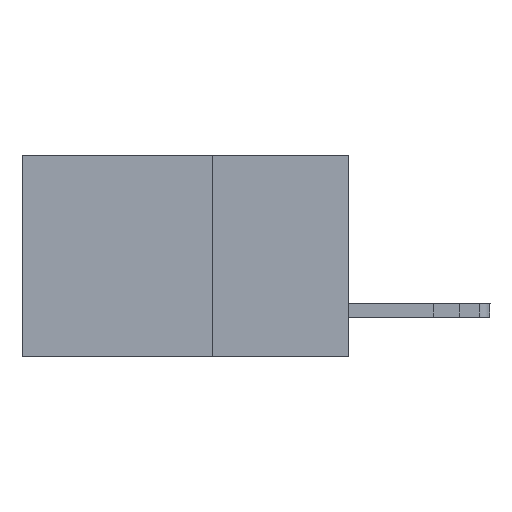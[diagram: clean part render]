
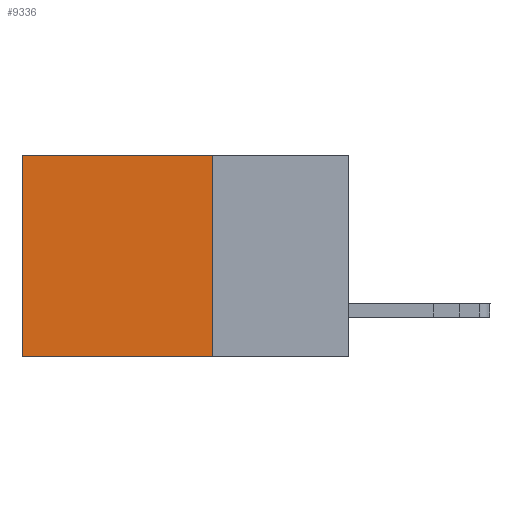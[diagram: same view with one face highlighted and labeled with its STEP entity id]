
A CAD part, left-side view. The second image highlights one B-rep face of the part: STEP entity #9336.
In plain terms, the highlighted planar face has unit normal (-1, 0, 0).
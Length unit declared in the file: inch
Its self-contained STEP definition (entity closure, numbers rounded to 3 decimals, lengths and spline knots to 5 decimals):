
#306 = LINE ( 'NONE', #15764, #18215 ) ;
#2104 = VECTOR ( 'NONE', #7133, 39.37008 ) ;
#2368 = LINE ( 'NONE', #3701, #2104 ) ;
#3596 = DIRECTION ( 'NONE',  ( 0., 1., 0. ) ) ;
#3701 = CARTESIAN_POINT ( 'NONE',  ( 0.298, 0.6, 0. ) ) ;
#3833 = AXIS2_PLACEMENT_3D ( 'NONE', #8523, #11875, #13608 ) ;
#5139 = EDGE_CURVE ( 'NONE', #19253, #16498, #306, .T. ) ;
#5282 = DIRECTION ( 'NONE',  ( 0., 1., 0. ) ) ;
#6829 = LINE ( 'NONE', #17029, #7639 ) ;
#7133 = DIRECTION ( 'NONE',  ( 0., 0., -1. ) ) ;
#7348 = EDGE_CURVE ( 'NONE', #20851, #14396, #19223, .T. ) ;
#7639 = VECTOR ( 'NONE', #13703, 39.37008 ) ;
#8523 = CARTESIAN_POINT ( 'NONE',  ( 0.298, 0.25, 0. ) ) ;
#8922 = CARTESIAN_POINT ( 'NONE',  ( 0.298, 0.25, 0. ) ) ;
#8927 = VECTOR ( 'NONE', #3596, 39.37008 ) ;
#9336 = ADVANCED_FACE ( 'NONE', ( #20766 ), #17016, .F. ) ;
#11068 = ORIENTED_EDGE ( 'NONE', *, *, #5139, .F. ) ;
#11875 = DIRECTION ( 'NONE',  ( 1., 0., 0. ) ) ;
#12524 = CARTESIAN_POINT ( 'NONE',  ( 0.298, 0.25, 0. ) ) ;
#13478 = ORIENTED_EDGE ( 'NONE', *, *, #19272, .T. ) ;
#13608 = DIRECTION ( 'NONE',  ( 0., 0., -1. ) ) ;
#13703 = DIRECTION ( 'NONE',  ( 0., 0., -1. ) ) ;
#14396 = VERTEX_POINT ( 'NONE', #18213 ) ;
#14557 = EDGE_LOOP ( 'NONE', ( #13478, #11068, #20999, #19009 ) ) ;
#14637 = EDGE_CURVE ( 'NONE', #20851, #19253, #6829, .T. ) ;
#15764 = CARTESIAN_POINT ( 'NONE',  ( 0.298, 0.25, -0.37 ) ) ;
#16102 = CARTESIAN_POINT ( 'NONE',  ( 0.298, 0.6, -0.37 ) ) ;
#16498 = VERTEX_POINT ( 'NONE', #16102 ) ;
#17016 = PLANE ( 'NONE',  #3833 ) ;
#17029 = CARTESIAN_POINT ( 'NONE',  ( 0.298, 0.25, 0. ) ) ;
#18213 = CARTESIAN_POINT ( 'NONE',  ( 0.298, 0.6, 0. ) ) ;
#18215 = VECTOR ( 'NONE', #5282, 39.37008 ) ;
#19009 = ORIENTED_EDGE ( 'NONE', *, *, #7348, .T. ) ;
#19223 = LINE ( 'NONE', #8922, #8927 ) ;
#19253 = VERTEX_POINT ( 'NONE', #21098 ) ;
#19272 = EDGE_CURVE ( 'NONE', #14396, #16498, #2368, .T. ) ;
#20766 = FACE_OUTER_BOUND ( 'NONE', #14557, .T. ) ;
#20851 = VERTEX_POINT ( 'NONE', #12524 ) ;
#20999 = ORIENTED_EDGE ( 'NONE', *, *, #14637, .F. ) ;
#21098 = CARTESIAN_POINT ( 'NONE',  ( 0.298, 0.25, -0.37 ) ) ;
